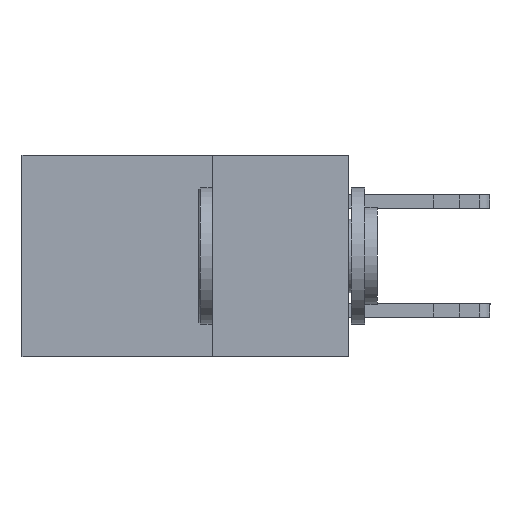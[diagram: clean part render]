
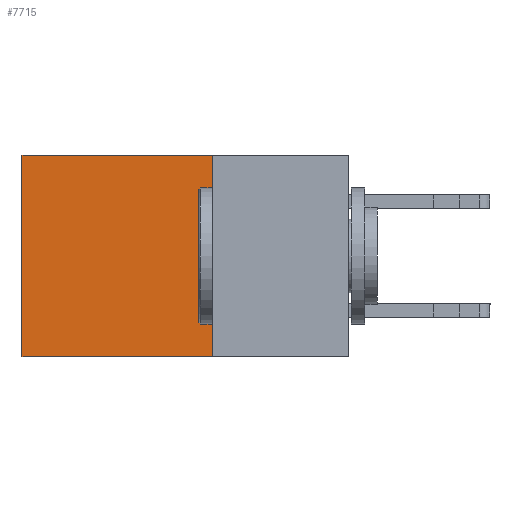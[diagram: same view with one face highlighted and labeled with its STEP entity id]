
A CAD part, left-side view. The second image highlights one B-rep face of the part: STEP entity #7715.
In plain terms, the highlighted planar face has unit normal (-1, 0, 0).
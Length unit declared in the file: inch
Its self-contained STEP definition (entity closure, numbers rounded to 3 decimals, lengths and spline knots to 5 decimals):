
#824 = CARTESIAN_POINT ( 'NONE',  ( 0.298, 0.25, 0. ) ) ;
#865 = LINE ( 'NONE', #12392, #2219 ) ;
#1093 = VERTEX_POINT ( 'NONE', #5623 ) ;
#1209 = VERTEX_POINT ( 'NONE', #2781 ) ;
#1279 = VECTOR ( 'NONE', #11268, 39.37008 ) ;
#1401 = VERTEX_POINT ( 'NONE', #6004 ) ;
#2133 = VECTOR ( 'NONE', #10466, 39.37008 ) ;
#2219 = VECTOR ( 'NONE', #2820, 39.37008 ) ;
#2465 = ORIENTED_EDGE ( 'NONE', *, *, #8599, .F. ) ;
#2781 = CARTESIAN_POINT ( 'NONE',  ( 0.298, 0.25, -0.37 ) ) ;
#2820 = DIRECTION ( 'NONE',  ( 0., 1., 0. ) ) ;
#2931 = EDGE_CURVE ( 'NONE', #1401, #7828, #9578, .T. ) ;
#3127 = CARTESIAN_POINT ( 'NONE',  ( 0.298, 0.25, 0. ) ) ;
#3847 = LINE ( 'NONE', #4204, #1279 ) ;
#3885 = DIRECTION ( 'NONE',  ( 0., 0., -1. ) ) ;
#4204 = CARTESIAN_POINT ( 'NONE',  ( 0.298, 0.25, -0.37 ) ) ;
#4205 = EDGE_CURVE ( 'NONE', #1093, #1209, #7559, .T. ) ;
#5623 = CARTESIAN_POINT ( 'NONE',  ( 0.298, 0.25, 0. ) ) ;
#5912 = DIRECTION ( 'NONE',  ( 0., 0., -1. ) ) ;
#6004 = CARTESIAN_POINT ( 'NONE',  ( 0.298, 0.6, 0. ) ) ;
#6881 = FACE_OUTER_BOUND ( 'NONE', #10471, .T. ) ;
#6884 = DIRECTION ( 'NONE',  ( 1., 0., 0. ) ) ;
#6963 = ORIENTED_EDGE ( 'NONE', *, *, #2931, .T. ) ;
#7116 = EDGE_CURVE ( 'NONE', #1093, #1401, #865, .T. ) ;
#7559 = LINE ( 'NONE', #824, #2133 ) ;
#7715 = ADVANCED_FACE ( 'NONE', ( #6881 ), #10691, .F. ) ;
#7736 = CARTESIAN_POINT ( 'NONE',  ( 0.298, 0.6, 0. ) ) ;
#7828 = VERTEX_POINT ( 'NONE', #10141 ) ;
#8306 = ORIENTED_EDGE ( 'NONE', *, *, #4205, .F. ) ;
#8599 = EDGE_CURVE ( 'NONE', #1209, #7828, #3847, .T. ) ;
#9578 = LINE ( 'NONE', #7736, #10010 ) ;
#10010 = VECTOR ( 'NONE', #3885, 39.37008 ) ;
#10141 = CARTESIAN_POINT ( 'NONE',  ( 0.298, 0.6, -0.37 ) ) ;
#10466 = DIRECTION ( 'NONE',  ( 0., 0., -1. ) ) ;
#10471 = EDGE_LOOP ( 'NONE', ( #6963, #2465, #8306, #11479 ) ) ;
#10691 = PLANE ( 'NONE',  #11052 ) ;
#11052 = AXIS2_PLACEMENT_3D ( 'NONE', #3127, #6884, #5912 ) ;
#11268 = DIRECTION ( 'NONE',  ( 0., 1., 0. ) ) ;
#11479 = ORIENTED_EDGE ( 'NONE', *, *, #7116, .T. ) ;
#12392 = CARTESIAN_POINT ( 'NONE',  ( 0.298, 0.25, 0. ) ) ;
